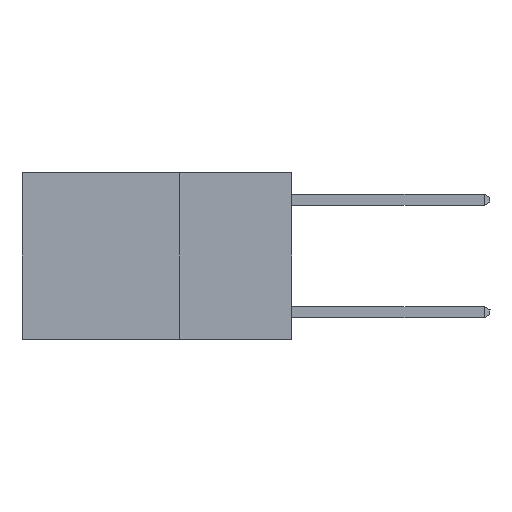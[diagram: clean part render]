
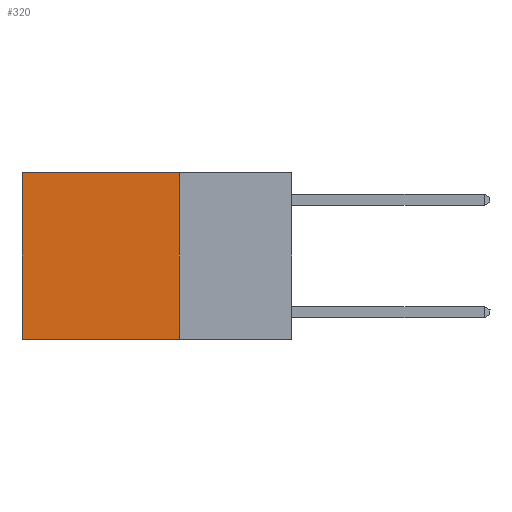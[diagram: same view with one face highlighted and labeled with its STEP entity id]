
A CAD part, left-side view. The second image highlights one B-rep face of the part: STEP entity #320.
In plain terms, the highlighted planar face has unit normal (-1, 0, 0).
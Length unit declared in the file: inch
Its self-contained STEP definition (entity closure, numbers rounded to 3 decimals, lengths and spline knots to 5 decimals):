
#177 = CARTESIAN_POINT ( 'NONE',  ( 0.2625, 0.6, -0.37 ) ) ;
#261 = DIRECTION ( 'NONE',  ( 0., 1., 0. ) ) ;
#286 = CARTESIAN_POINT ( 'NONE',  ( 0.2625, 0.25, -0.37 ) ) ;
#320 = ADVANCED_FACE ( 'NONE', ( #697 ), #4097, .F. ) ;
#697 = FACE_OUTER_BOUND ( 'NONE', #1004, .T. ) ;
#908 = LINE ( 'NONE', #2199, #2783 ) ;
#920 = DIRECTION ( 'NONE',  ( 1., 0., 0. ) ) ;
#1004 = EDGE_LOOP ( 'NONE', ( #2949, #3180, #5403, #9052 ) ) ;
#1036 = EDGE_CURVE ( 'NONE', #2807, #4157, #8836, .T. ) ;
#1180 = CARTESIAN_POINT ( 'NONE',  ( 0.2625, 0.25, 0. ) ) ;
#1541 = DIRECTION ( 'NONE',  ( 0., 0., -1. ) ) ;
#1961 = VERTEX_POINT ( 'NONE', #4360 ) ;
#2082 = EDGE_CURVE ( 'NONE', #4157, #5921, #7399, .T. ) ;
#2189 = DIRECTION ( 'NONE',  ( 0., 0., -1. ) ) ;
#2199 = CARTESIAN_POINT ( 'NONE',  ( 0.2625, 0.25, 0. ) ) ;
#2557 = EDGE_CURVE ( 'NONE', #2807, #1961, #908, .T. ) ;
#2783 = VECTOR ( 'NONE', #2189, 39.37008 ) ;
#2807 = VERTEX_POINT ( 'NONE', #1180 ) ;
#2949 = ORIENTED_EDGE ( 'NONE', *, *, #2082, .T. ) ;
#2969 = EDGE_CURVE ( 'NONE', #1961, #5921, #4343, .T. ) ;
#3003 = DIRECTION ( 'NONE',  ( 0., 1., 0. ) ) ;
#3138 = CARTESIAN_POINT ( 'NONE',  ( 0.2625, 0.25, 0. ) ) ;
#3180 = ORIENTED_EDGE ( 'NONE', *, *, #2969, .F. ) ;
#3411 = VECTOR ( 'NONE', #3003, 39.37008 ) ;
#4019 = DIRECTION ( 'NONE',  ( 0., 0., -1. ) ) ;
#4038 = CARTESIAN_POINT ( 'NONE',  ( 0.2625, 0.6, 0. ) ) ;
#4042 = CARTESIAN_POINT ( 'NONE',  ( 0.2625, 0.25, 0. ) ) ;
#4097 = PLANE ( 'NONE',  #7701 ) ;
#4141 = VECTOR ( 'NONE', #261, 39.37008 ) ;
#4157 = VERTEX_POINT ( 'NONE', #6677 ) ;
#4343 = LINE ( 'NONE', #286, #4141 ) ;
#4360 = CARTESIAN_POINT ( 'NONE',  ( 0.2625, 0.25, -0.37 ) ) ;
#5403 = ORIENTED_EDGE ( 'NONE', *, *, #2557, .F. ) ;
#5578 = VECTOR ( 'NONE', #4019, 39.37008 ) ;
#5921 = VERTEX_POINT ( 'NONE', #177 ) ;
#6677 = CARTESIAN_POINT ( 'NONE',  ( 0.2625, 0.6, 0. ) ) ;
#7399 = LINE ( 'NONE', #4038, #5578 ) ;
#7701 = AXIS2_PLACEMENT_3D ( 'NONE', #4042, #920, #1541 ) ;
#8836 = LINE ( 'NONE', #3138, #3411 ) ;
#9052 = ORIENTED_EDGE ( 'NONE', *, *, #1036, .T. ) ;
